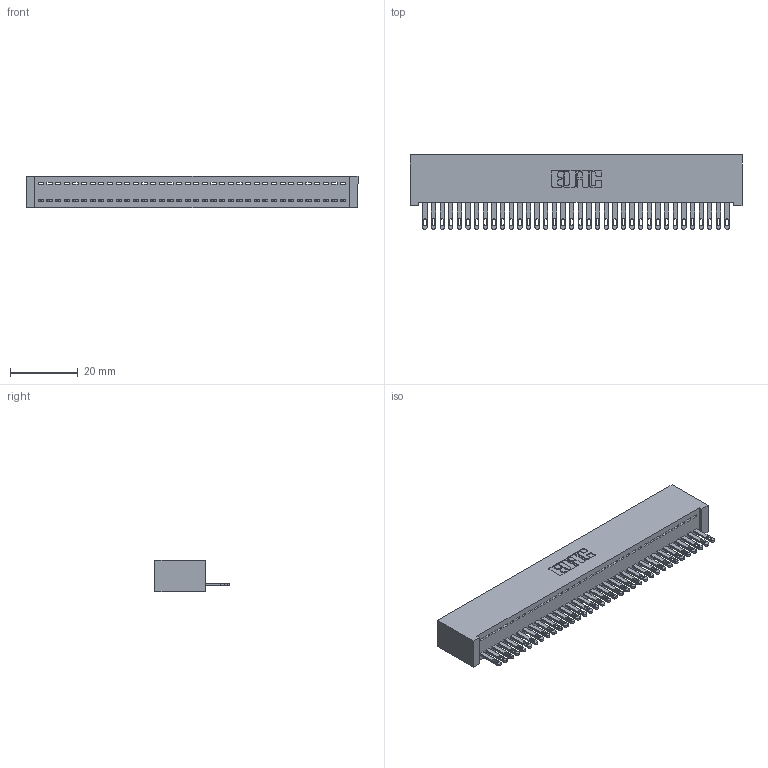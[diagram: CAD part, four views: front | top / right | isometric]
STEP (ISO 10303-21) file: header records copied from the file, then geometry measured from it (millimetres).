
FILE_DESCRIPTION (( 'STEP AP203' ), '1' );
FILE_NAME ('342-036-500-101.STEP', '2018-08-11T19:44:27', ( '' ), ( '' ), 'SwSTEP 2.0', 'SolidWorks 2016', '' );
FILE_SCHEMA (( 'CONFIG_CONTROL_DESIGN' ));
Length unit declared in the file: inch
Products named in the file (3): 342 Part_Lugless; 345-292-001_345-293-100; 342-036-500-101
Assembly tree (37 placements, depth 2):
  342-036-500-101
    342 Part_Lugless
    345-292-001_345-293-100  x36
Bounding box: 97.69 x 21.85 x 9.4 mm (x, y, z)
Volume: 8974.5 mm3; surface area: 13460.7 mm2
Topology: 37 solids, 37 shells, 2046 faces, 6323 edges, 4214 vertices
Faces by surface type: plane 1358, cylinder 688
Entity records: 22305 total; most frequent: CARTESIAN_POINT 3854, ORIENTED_EDGE 3826, DIRECTION 3257, EDGE_CURVE 1913, LINE 1789, VECTOR 1789, VERTEX_POINT 1274, AXIS2_PLACEMENT_3D 734
